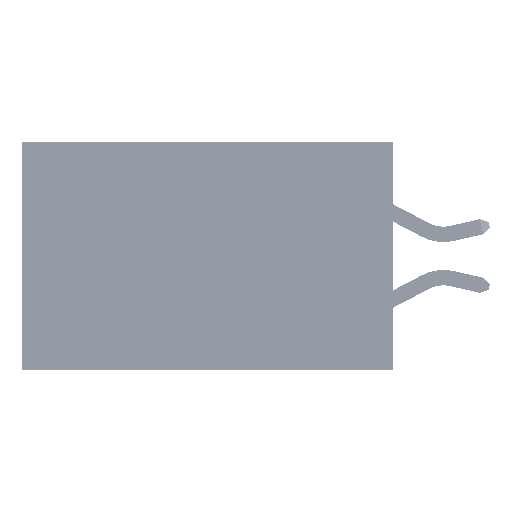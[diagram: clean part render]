
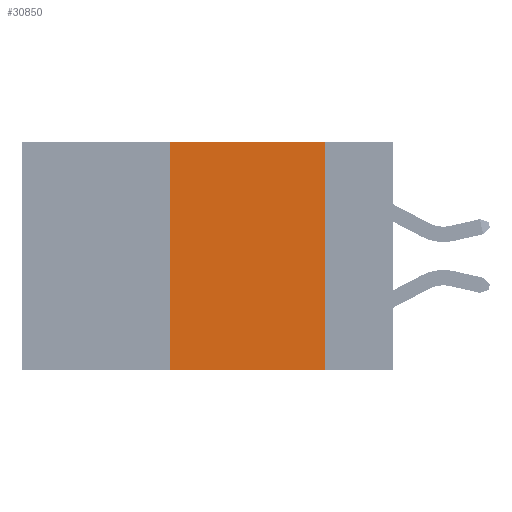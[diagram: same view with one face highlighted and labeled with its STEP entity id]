
A CAD part, left-side view. The second image highlights one B-rep face of the part: STEP entity #30850.
In plain terms, the highlighted planar face has unit normal (-1, 0, 0).
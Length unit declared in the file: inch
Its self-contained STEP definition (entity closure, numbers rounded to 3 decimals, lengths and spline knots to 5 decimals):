
#3153 = CARTESIAN_POINT ( 'NONE',  ( 0., 0.36, 0. ) ) ;
#5243 = EDGE_CURVE ( 'NONE', #43771, #34870, #14286, .T. ) ;
#5842 = DIRECTION ( 'NONE',  ( 1., 0., 0. ) ) ;
#8114 = EDGE_LOOP ( 'NONE', ( #36163, #52515, #11974, #23645 ) ) ;
#8128 = VECTOR ( 'NONE', #10143, 39.37008 ) ;
#9050 = CARTESIAN_POINT ( 'NONE',  ( 0., 0.6, 0. ) ) ;
#10143 = DIRECTION ( 'NONE',  ( 0., 0., 1. ) ) ;
#10663 = CARTESIAN_POINT ( 'NONE',  ( 0., 0.11, 0. ) ) ;
#10689 = EDGE_CURVE ( 'NONE', #43771, #46076, #51531, .T. ) ;
#11974 = ORIENTED_EDGE ( 'NONE', *, *, #10689, .F. ) ;
#12962 = DIRECTION ( 'NONE',  ( 0., -1., 0. ) ) ;
#14286 = LINE ( 'NONE', #52289, #48672 ) ;
#15914 = DIRECTION ( 'NONE',  ( 0., -1., 0. ) ) ;
#17084 = CARTESIAN_POINT ( 'NONE',  ( 0., 0.6, 0. ) ) ;
#18663 = DIRECTION ( 'NONE',  ( 0., 0., -1. ) ) ;
#19157 = CARTESIAN_POINT ( 'NONE',  ( 0., 0.11, 0. ) ) ;
#19432 = VECTOR ( 'NONE', #39253, 39.37008 ) ;
#19642 = EDGE_CURVE ( 'NONE', #46076, #27731, #31556, .T. ) ;
#23645 = ORIENTED_EDGE ( 'NONE', *, *, #5243, .T. ) ;
#24399 = AXIS2_PLACEMENT_3D ( 'NONE', #9050, #5842, #18663 ) ;
#26427 = CARTESIAN_POINT ( 'NONE',  ( 0., 0.36, 0. ) ) ;
#27731 = VERTEX_POINT ( 'NONE', #19157 ) ;
#29643 = VECTOR ( 'NONE', #12962, 39.37008 ) ;
#30132 = PLANE ( 'NONE',  #24399 ) ;
#30850 = ADVANCED_FACE ( 'NONE', ( #40174 ), #30132, .F. ) ;
#31556 = LINE ( 'NONE', #17084, #29643 ) ;
#31909 = CARTESIAN_POINT ( 'NONE',  ( 0., 0.36, -0.37 ) ) ;
#34870 = VERTEX_POINT ( 'NONE', #44813 ) ;
#36163 = ORIENTED_EDGE ( 'NONE', *, *, #49223, .F. ) ;
#39253 = DIRECTION ( 'NONE',  ( 0., 0., -1. ) ) ;
#40174 = FACE_OUTER_BOUND ( 'NONE', #8114, .T. ) ;
#43771 = VERTEX_POINT ( 'NONE', #31909 ) ;
#44813 = CARTESIAN_POINT ( 'NONE',  ( 0., 0.11, -0.37 ) ) ;
#46076 = VERTEX_POINT ( 'NONE', #3153 ) ;
#47543 = LINE ( 'NONE', #10663, #19432 ) ;
#48672 = VECTOR ( 'NONE', #15914, 39.37008 ) ;
#49223 = EDGE_CURVE ( 'NONE', #27731, #34870, #47543, .T. ) ;
#51531 = LINE ( 'NONE', #26427, #8128 ) ;
#52289 = CARTESIAN_POINT ( 'NONE',  ( 0., 0.6, -0.37 ) ) ;
#52515 = ORIENTED_EDGE ( 'NONE', *, *, #19642, .F. ) ;
